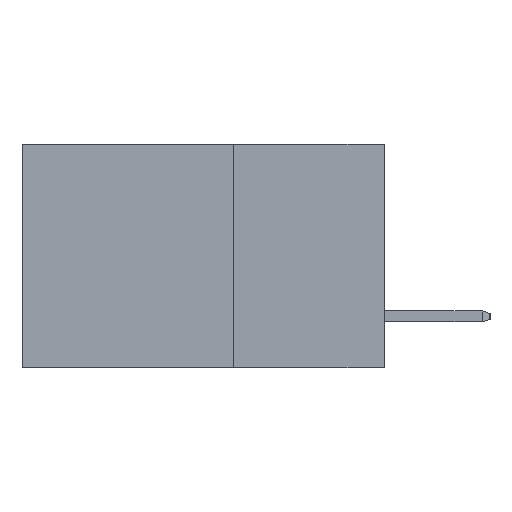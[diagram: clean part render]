
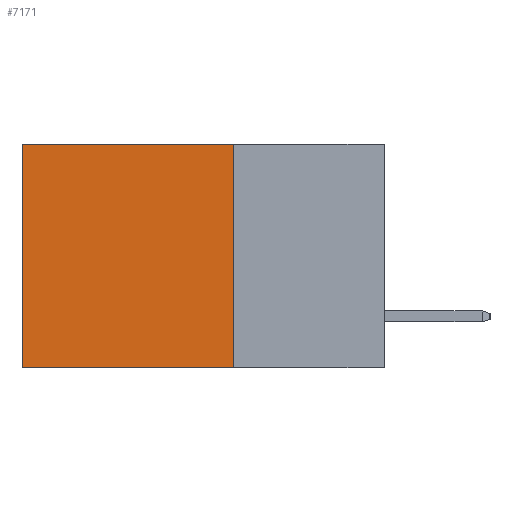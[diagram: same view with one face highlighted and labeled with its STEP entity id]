
A CAD part, left-side view. The second image highlights one B-rep face of the part: STEP entity #7171.
In plain terms, the highlighted planar face has unit normal (-1, 0, 0).
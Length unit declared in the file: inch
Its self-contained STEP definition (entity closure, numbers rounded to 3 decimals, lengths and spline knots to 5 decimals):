
#1565 = VECTOR ( 'NONE', #3848, 39.37008 ) ;
#2109 = CARTESIAN_POINT ( 'NONE',  ( 0.2615, 0.25, -0.37 ) ) ;
#3092 = DIRECTION ( 'NONE',  ( 0., 0., -1. ) ) ;
#3213 = CARTESIAN_POINT ( 'NONE',  ( 0.2615, 0.6, -0.37 ) ) ;
#3548 = VERTEX_POINT ( 'NONE', #10130 ) ;
#3718 = ORIENTED_EDGE ( 'NONE', *, *, #10672, .F. ) ;
#3848 = DIRECTION ( 'NONE',  ( 0., 1., 0. ) ) ;
#4625 = AXIS2_PLACEMENT_3D ( 'NONE', #7259, #7231, #7149 ) ;
#4665 = LINE ( 'NONE', #2109, #1565 ) ;
#4796 = VECTOR ( 'NONE', #6590, 39.37008 ) ;
#5718 = CARTESIAN_POINT ( 'NONE',  ( 0.2615, 0.25, -0.37 ) ) ;
#5889 = CARTESIAN_POINT ( 'NONE',  ( 0.2615, 0.25, -0.37 ) ) ;
#6021 = CARTESIAN_POINT ( 'NONE',  ( 0.2615, 0.6, 0. ) ) ;
#6449 = LINE ( 'NONE', #8884, #11167 ) ;
#6590 = DIRECTION ( 'NONE',  ( 0., 0., -1. ) ) ;
#6722 = EDGE_CURVE ( 'NONE', #7242, #3548, #10334, .T. ) ;
#7149 = DIRECTION ( 'NONE',  ( 0., 0., -1. ) ) ;
#7171 = ADVANCED_FACE ( 'NONE', ( #10325 ), #7399, .F. ) ;
#7231 = DIRECTION ( 'NONE',  ( 1., 0., 0. ) ) ;
#7242 = VERTEX_POINT ( 'NONE', #6021 ) ;
#7247 = VERTEX_POINT ( 'NONE', #5889 ) ;
#7259 = CARTESIAN_POINT ( 'NONE',  ( 0.2615, 0.25, -0.37 ) ) ;
#7399 = PLANE ( 'NONE',  #4625 ) ;
#7555 = CARTESIAN_POINT ( 'NONE',  ( 0.2615, 0.25, 0. ) ) ;
#7868 = EDGE_LOOP ( 'NONE', ( #9302, #10158, #3718, #8881 ) ) ;
#7939 = VECTOR ( 'NONE', #3092, 39.37008 ) ;
#8261 = EDGE_CURVE ( 'NONE', #10764, #7242, #6449, .T. ) ;
#8844 = DIRECTION ( 'NONE',  ( 0., 1., 0. ) ) ;
#8881 = ORIENTED_EDGE ( 'NONE', *, *, #8261, .T. ) ;
#8884 = CARTESIAN_POINT ( 'NONE',  ( 0.2615, 0.25, 0. ) ) ;
#9302 = ORIENTED_EDGE ( 'NONE', *, *, #6722, .T. ) ;
#10130 = CARTESIAN_POINT ( 'NONE',  ( 0.2615, 0.6, -0.37 ) ) ;
#10158 = ORIENTED_EDGE ( 'NONE', *, *, #10522, .F. ) ;
#10325 = FACE_OUTER_BOUND ( 'NONE', #7868, .T. ) ;
#10334 = LINE ( 'NONE', #3213, #7939 ) ;
#10522 = EDGE_CURVE ( 'NONE', #7247, #3548, #4665, .T. ) ;
#10672 = EDGE_CURVE ( 'NONE', #10764, #7247, #11237, .T. ) ;
#10764 = VERTEX_POINT ( 'NONE', #7555 ) ;
#11167 = VECTOR ( 'NONE', #8844, 39.37008 ) ;
#11237 = LINE ( 'NONE', #5718, #4796 ) ;
